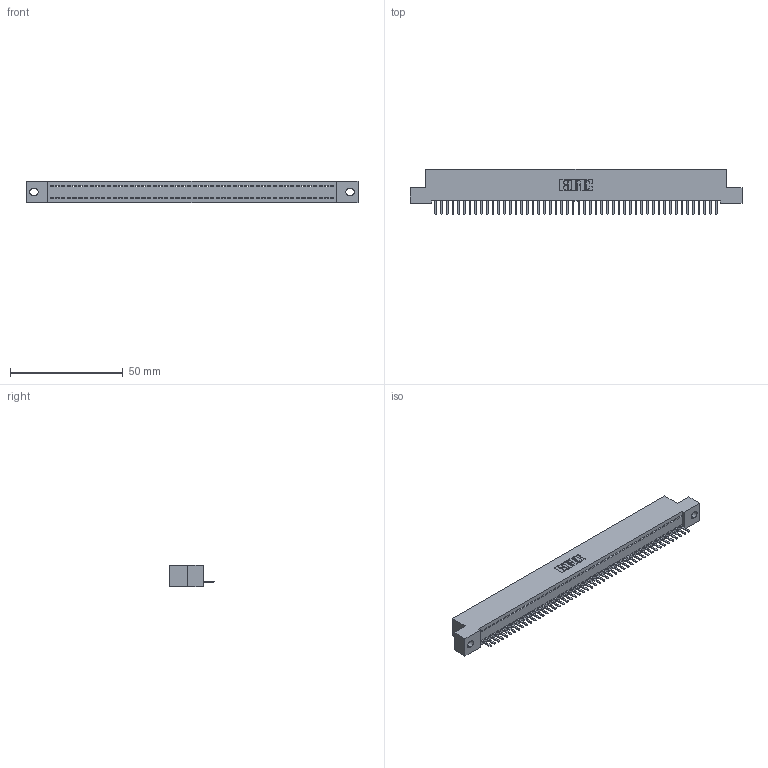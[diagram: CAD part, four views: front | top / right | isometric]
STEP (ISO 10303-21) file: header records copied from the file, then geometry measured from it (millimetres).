
FILE_DESCRIPTION (( 'STEP AP203' ), '1' );
FILE_NAME ('392-050-520-102.STEP', '2018-08-17T00:45:51', ( '' ), ( '' ), 'SwSTEP 2.0', 'SolidWorks 2016', '' );
FILE_SCHEMA (( 'CONFIG_CONTROL_DESIGN' ));
Length unit declared in the file: inch
Products named in the file (3): 342 Part_.128 Slot; 345-292-001_345-293-120; 392-050-520-102
Assembly tree (51 placements, depth 2):
  392-050-520-102
    342 Part_.128 Slot
    345-292-001_345-293-120  x50
Bounding box: 147.32 x 20.02 x 9.4 mm (x, y, z)
Volume: 12750.5 mm3; surface area: 18172.6 mm2
Topology: 51 solids, 51 shells, 3214 faces, 9511 edges, 6206 vertices
Faces by surface type: plane 2270, cylinder 944
Entity records: 29649 total; most frequent: CARTESIAN_POINT 5132, ORIENTED_EDGE 5106, DIRECTION 4301, EDGE_CURVE 2553, VECTOR 2421, LINE 2421, VERTEX_POINT 1698, AXIS2_PLACEMENT_3D 940
